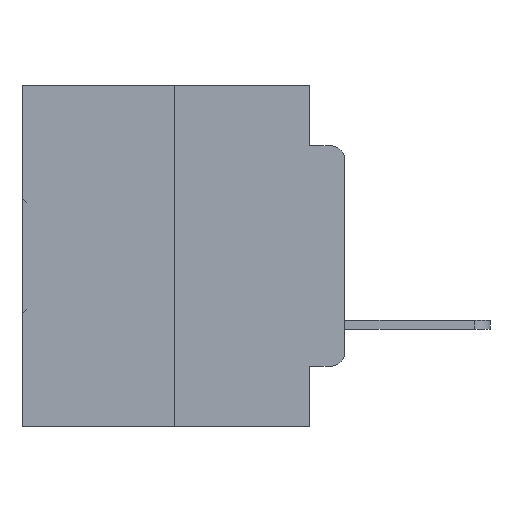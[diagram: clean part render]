
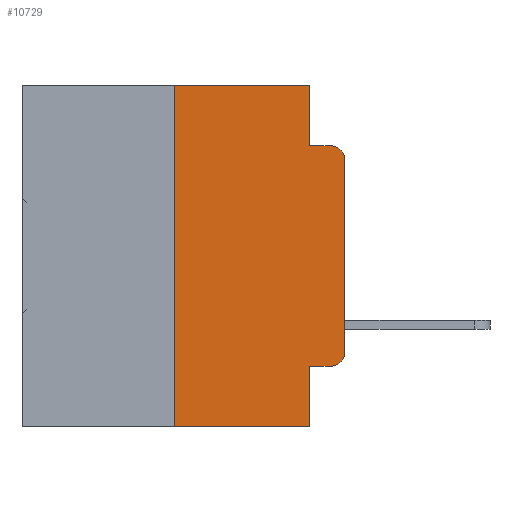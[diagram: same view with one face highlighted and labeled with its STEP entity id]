
A CAD part, left-side view. The second image highlights one B-rep face of the part: STEP entity #10729.
In plain terms, the highlighted planar face has unit normal (-1, 0, 0).
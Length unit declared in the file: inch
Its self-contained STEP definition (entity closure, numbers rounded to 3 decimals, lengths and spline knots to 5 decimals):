
#45 = CARTESIAN_POINT ( 'NONE',  ( 0., 0.051, -0.0885 ) ) ;
#1632 = CARTESIAN_POINT ( 'NONE',  ( 0., 0.051, 0. ) ) ;
#2194 = LINE ( 'NONE', #18005, #15825 ) ;
#2756 = PLANE ( 'NONE',  #27935 ) ;
#2757 = CARTESIAN_POINT ( 'NONE',  ( 0., 0., 0. ) ) ;
#3042 = ORIENTED_EDGE ( 'NONE', *, *, #11930, .T. ) ;
#3439 = CARTESIAN_POINT ( 'NONE',  ( 0., 0.051, -0.0885 ) ) ;
#3720 = CIRCLE ( 'NONE', #12909, 0.02 ) ;
#4156 = VERTEX_POINT ( 'NONE', #22129 ) ;
#4902 = VERTEX_POINT ( 'NONE', #17250 ) ;
#5509 = CARTESIAN_POINT ( 'NONE',  ( 0., 0.473, 0. ) ) ;
#5556 = VERTEX_POINT ( 'NONE', #29323 ) ;
#5824 = CARTESIAN_POINT ( 'NONE',  ( 0., 0.02, -0.4115 ) ) ;
#6424 = EDGE_CURVE ( 'NONE', #26583, #12985, #29467, .T. ) ;
#6811 = CARTESIAN_POINT ( 'NONE',  ( 0., 0.051, -0.4115 ) ) ;
#7803 = FACE_OUTER_BOUND ( 'NONE', #7905, .T. ) ;
#7905 = EDGE_LOOP ( 'NONE', ( #3042, #9158, #11680, #12404, #14064, #15890, #23332, #25886, #26566, #27452 ) ) ;
#8258 = EDGE_CURVE ( 'NONE', #12985, #4156, #17719, .T. ) ;
#8267 = DIRECTION ( 'NONE',  ( 0., 0., -1. ) ) ;
#9037 = VECTOR ( 'NONE', #16651, 39.37008 ) ;
#9120 = VERTEX_POINT ( 'NONE', #22771 ) ;
#9158 = ORIENTED_EDGE ( 'NONE', *, *, #15504, .T. ) ;
#10080 = DIRECTION ( 'NONE',  ( -1., 0., 0. ) ) ;
#10116 = DIRECTION ( 'NONE',  ( 0., 0., -1. ) ) ;
#10219 = CARTESIAN_POINT ( 'NONE',  ( 0., 0.25, -0.5 ) ) ;
#10342 = CARTESIAN_POINT ( 'NONE',  ( 0., 0.051, -0.4115 ) ) ;
#10593 = VERTEX_POINT ( 'NONE', #10219 ) ;
#10631 = CARTESIAN_POINT ( 'NONE',  ( 0., 0.02, -0.1085 ) ) ;
#10651 = EDGE_CURVE ( 'NONE', #10593, #5556, #11262, .T. ) ;
#10729 = ADVANCED_FACE ( 'NONE', ( #7803 ), #2756, .F. ) ;
#11262 = LINE ( 'NONE', #30718, #25058 ) ;
#11578 = CIRCLE ( 'NONE', #12079, 0.02 ) ;
#11680 = ORIENTED_EDGE ( 'NONE', *, *, #8258, .F. ) ;
#11930 = EDGE_CURVE ( 'NONE', #9120, #32658, #13707, .T. ) ;
#12079 = AXIS2_PLACEMENT_3D ( 'NONE', #25652, #10080, #28034 ) ;
#12404 = ORIENTED_EDGE ( 'NONE', *, *, #6424, .F. ) ;
#12780 = VECTOR ( 'NONE', #24856, 39.37008 ) ;
#12909 = AXIS2_PLACEMENT_3D ( 'NONE', #10631, #28493, #13322 ) ;
#12985 = VERTEX_POINT ( 'NONE', #3439 ) ;
#13322 = DIRECTION ( 'NONE',  ( 0., 0., -1. ) ) ;
#13707 = LINE ( 'NONE', #2757, #27294 ) ;
#14064 = ORIENTED_EDGE ( 'NONE', *, *, #27147, .F. ) ;
#14978 = DIRECTION ( 'NONE',  ( 0., -1., 0. ) ) ;
#15504 = EDGE_CURVE ( 'NONE', #32658, #4156, #3720, .T. ) ;
#15825 = VECTOR ( 'NONE', #18122, 39.37008 ) ;
#15890 = ORIENTED_EDGE ( 'NONE', *, *, #32467, .F. ) ;
#15940 = DIRECTION ( 'NONE',  ( 0., -1., 0. ) ) ;
#16651 = DIRECTION ( 'NONE',  ( 0., 0., -1. ) ) ;
#17250 = CARTESIAN_POINT ( 'NONE',  ( 0., 0.25, 0. ) ) ;
#17719 = LINE ( 'NONE', #45, #24458 ) ;
#17906 = VECTOR ( 'NONE', #10116, 39.37008 ) ;
#17977 = LINE ( 'NONE', #6811, #23922 ) ;
#18005 = CARTESIAN_POINT ( 'NONE',  ( 0., 0.473, 0. ) ) ;
#18122 = DIRECTION ( 'NONE',  ( 0., -1., 0. ) ) ;
#18705 = CARTESIAN_POINT ( 'NONE',  ( 0., 0.051, 0. ) ) ;
#18968 = EDGE_CURVE ( 'NONE', #25493, #9120, #11578, .T. ) ;
#19778 = CARTESIAN_POINT ( 'NONE',  ( 0., 0.25, 0. ) ) ;
#20812 = CARTESIAN_POINT ( 'NONE',  ( 0., 0.051, 0. ) ) ;
#21465 = DIRECTION ( 'NONE',  ( 0., 0., 1. ) ) ;
#22129 = CARTESIAN_POINT ( 'NONE',  ( 0., 0.02, -0.0885 ) ) ;
#22771 = CARTESIAN_POINT ( 'NONE',  ( 0., 0., -0.3915 ) ) ;
#23332 = ORIENTED_EDGE ( 'NONE', *, *, #10651, .T. ) ;
#23922 = VECTOR ( 'NONE', #14978, 39.37008 ) ;
#23993 = DIRECTION ( 'NONE',  ( 1., 0., 0. ) ) ;
#24458 = VECTOR ( 'NONE', #26638, 39.37008 ) ;
#24646 = LINE ( 'NONE', #1632, #17906 ) ;
#24856 = DIRECTION ( 'NONE',  ( 0., 0., 1. ) ) ;
#25058 = VECTOR ( 'NONE', #15940, 39.37008 ) ;
#25493 = VERTEX_POINT ( 'NONE', #5824 ) ;
#25652 = CARTESIAN_POINT ( 'NONE',  ( 0., 0.02, -0.3915 ) ) ;
#25743 = EDGE_CURVE ( 'NONE', #29043, #25493, #17977, .T. ) ;
#25886 = ORIENTED_EDGE ( 'NONE', *, *, #28912, .F. ) ;
#26566 = ORIENTED_EDGE ( 'NONE', *, *, #25743, .T. ) ;
#26583 = VERTEX_POINT ( 'NONE', #20812 ) ;
#26638 = DIRECTION ( 'NONE',  ( 0., -1., 0. ) ) ;
#27147 = EDGE_CURVE ( 'NONE', #4902, #26583, #2194, .T. ) ;
#27294 = VECTOR ( 'NONE', #21465, 39.37008 ) ;
#27452 = ORIENTED_EDGE ( 'NONE', *, *, #18968, .T. ) ;
#27935 = AXIS2_PLACEMENT_3D ( 'NONE', #5509, #23993, #8267 ) ;
#28034 = DIRECTION ( 'NONE',  ( 0., 0., -1. ) ) ;
#28493 = DIRECTION ( 'NONE',  ( -1., 0., 0. ) ) ;
#28912 = EDGE_CURVE ( 'NONE', #29043, #5556, #24646, .T. ) ;
#29043 = VERTEX_POINT ( 'NONE', #10342 ) ;
#29323 = CARTESIAN_POINT ( 'NONE',  ( 0., 0.051, -0.5 ) ) ;
#29467 = LINE ( 'NONE', #18705, #9037 ) ;
#30718 = CARTESIAN_POINT ( 'NONE',  ( 0., 0.473, -0.5 ) ) ;
#32050 = CARTESIAN_POINT ( 'NONE',  ( 0., 0., -0.1085 ) ) ;
#32467 = EDGE_CURVE ( 'NONE', #10593, #4902, #32473, .T. ) ;
#32473 = LINE ( 'NONE', #19778, #12780 ) ;
#32658 = VERTEX_POINT ( 'NONE', #32050 ) ;
